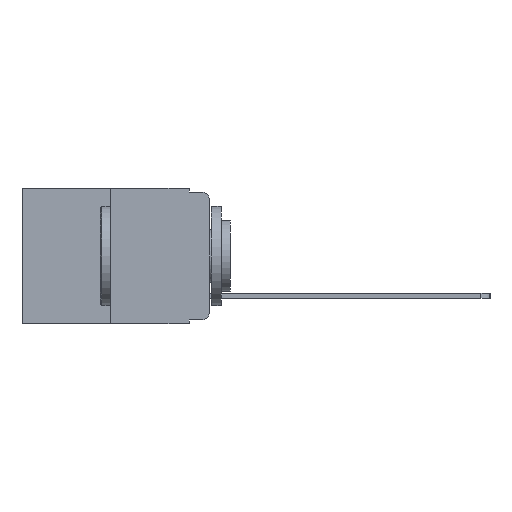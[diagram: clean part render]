
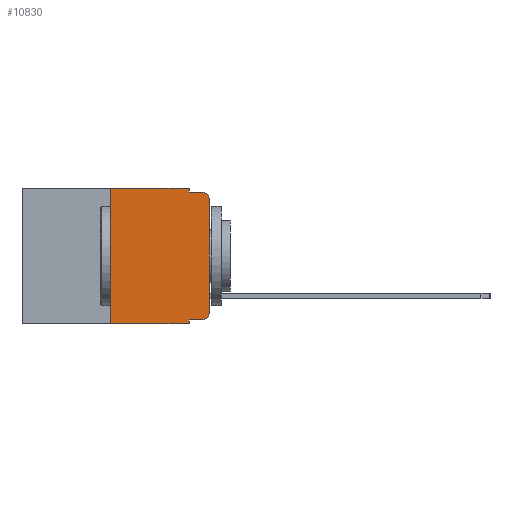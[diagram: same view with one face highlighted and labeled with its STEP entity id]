
A CAD part, left-side view. The second image highlights one B-rep face of the part: STEP entity #10830.
In plain terms, the highlighted planar face has unit normal (-1, 0, 0).
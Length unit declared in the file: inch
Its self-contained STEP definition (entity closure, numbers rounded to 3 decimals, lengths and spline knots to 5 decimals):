
#8 = CARTESIAN_POINT ( 'NONE',  ( 0., 0.051, 0. ) ) ;
#132 = CARTESIAN_POINT ( 'NONE',  ( 0., 0.25, -0.343 ) ) ;
#221 = VERTEX_POINT ( 'NONE', #3961 ) ;
#240 = LINE ( 'NONE', #15328, #3364 ) ;
#685 = VERTEX_POINT ( 'NONE', #11885 ) ;
#1372 = CARTESIAN_POINT ( 'NONE',  ( 0., 0.051, -0.01 ) ) ;
#1653 = ORIENTED_EDGE ( 'NONE', *, *, #17559, .T. ) ;
#2382 = VERTEX_POINT ( 'NONE', #10054 ) ;
#2571 = DIRECTION ( 'NONE',  ( 0., 0., -1. ) ) ;
#2594 = DIRECTION ( 'NONE',  ( 0., -1., 0. ) ) ;
#2757 = FACE_OUTER_BOUND ( 'NONE', #11270, .T. ) ;
#2986 = CARTESIAN_POINT ( 'NONE',  ( 0., 0.02, -0.313 ) ) ;
#3223 = DIRECTION ( 'NONE',  ( 0., 0., 1. ) ) ;
#3364 = VECTOR ( 'NONE', #18059, 39.37008 ) ;
#3961 = CARTESIAN_POINT ( 'NONE',  ( 0., 0., -0.313 ) ) ;
#4493 = DIRECTION ( 'NONE',  ( 0., 0., -1. ) ) ;
#4550 = VECTOR ( 'NONE', #17409, 39.37008 ) ;
#4647 = VERTEX_POINT ( 'NONE', #8 ) ;
#4823 = CARTESIAN_POINT ( 'NONE',  ( 0., 0.051, -0.333 ) ) ;
#5031 = CARTESIAN_POINT ( 'NONE',  ( 0., 0.473, 0. ) ) ;
#5142 = CIRCLE ( 'NONE', #14515, 0.02 ) ;
#5199 = VERTEX_POINT ( 'NONE', #7287 ) ;
#5489 = EDGE_CURVE ( 'NONE', #8750, #4647, #18431, .T. ) ;
#5506 = VECTOR ( 'NONE', #12727, 39.37008 ) ;
#5660 = ORIENTED_EDGE ( 'NONE', *, *, #14820, .F. ) ;
#6102 = ORIENTED_EDGE ( 'NONE', *, *, #5489, .F. ) ;
#6231 = CARTESIAN_POINT ( 'NONE',  ( 0., 0.051, 0. ) ) ;
#6409 = VERTEX_POINT ( 'NONE', #1372 ) ;
#6485 = LINE ( 'NONE', #9879, #17194 ) ;
#6561 = LINE ( 'NONE', #15604, #17689 ) ;
#6562 = ORIENTED_EDGE ( 'NONE', *, *, #12995, .F. ) ;
#6955 = VERTEX_POINT ( 'NONE', #4823 ) ;
#7062 = LINE ( 'NONE', #10476, #18149 ) ;
#7098 = CARTESIAN_POINT ( 'NONE',  ( 0., 0.25, 0. ) ) ;
#7259 = DIRECTION ( 'NONE',  ( -1., 0., 0. ) ) ;
#7287 = CARTESIAN_POINT ( 'NONE',  ( 0., 0., -0.03 ) ) ;
#7500 = ORIENTED_EDGE ( 'NONE', *, *, #9250, .T. ) ;
#7564 = VERTEX_POINT ( 'NONE', #132 ) ;
#8093 = CIRCLE ( 'NONE', #16236, 0.02 ) ;
#8441 = LINE ( 'NONE', #6231, #4550 ) ;
#8595 = AXIS2_PLACEMENT_3D ( 'NONE', #9854, #11267, #2571 ) ;
#8750 = VERTEX_POINT ( 'NONE', #10559 ) ;
#9063 = ORIENTED_EDGE ( 'NONE', *, *, #18463, .T. ) ;
#9250 = EDGE_CURVE ( 'NONE', #2382, #221, #8093, .T. ) ;
#9365 = LINE ( 'NONE', #7098, #5506 ) ;
#9854 = CARTESIAN_POINT ( 'NONE',  ( 0., 0.473, 0. ) ) ;
#9879 = CARTESIAN_POINT ( 'NONE',  ( 0., 0.051, -0.333 ) ) ;
#10054 = CARTESIAN_POINT ( 'NONE',  ( 0., 0.02, -0.333 ) ) ;
#10202 = EDGE_CURVE ( 'NONE', #6955, #2382, #6485, .T. ) ;
#10476 = CARTESIAN_POINT ( 'NONE',  ( 0., 0., 0. ) ) ;
#10559 = CARTESIAN_POINT ( 'NONE',  ( 0., 0.25, 0. ) ) ;
#10817 = ORIENTED_EDGE ( 'NONE', *, *, #10202, .T. ) ;
#10830 = ADVANCED_FACE ( 'NONE', ( #2757 ), #12592, .F. ) ;
#11126 = VECTOR ( 'NONE', #13601, 39.37008 ) ;
#11267 = DIRECTION ( 'NONE',  ( 1., 0., 0. ) ) ;
#11270 = EDGE_LOOP ( 'NONE', ( #9063, #1653, #5660, #16848, #6102, #6562, #14077, #17690, #10817, #7500 ) ) ;
#11885 = CARTESIAN_POINT ( 'NONE',  ( 0., 0.02, -0.01 ) ) ;
#12034 = EDGE_CURVE ( 'NONE', #6955, #14273, #17162, .T. ) ;
#12592 = PLANE ( 'NONE',  #8595 ) ;
#12727 = DIRECTION ( 'NONE',  ( 0., 0., 1. ) ) ;
#12995 = EDGE_CURVE ( 'NONE', #7564, #8750, #9365, .T. ) ;
#13060 = DIRECTION ( 'NONE',  ( -1., 0., 0. ) ) ;
#13540 = VECTOR ( 'NONE', #17748, 39.37008 ) ;
#13601 = DIRECTION ( 'NONE',  ( 0., -1., 0. ) ) ;
#13902 = EDGE_CURVE ( 'NONE', #4647, #6409, #8441, .T. ) ;
#14077 = ORIENTED_EDGE ( 'NONE', *, *, #14148, .T. ) ;
#14148 = EDGE_CURVE ( 'NONE', #7564, #14273, #240, .T. ) ;
#14273 = VERTEX_POINT ( 'NONE', #15686 ) ;
#14515 = AXIS2_PLACEMENT_3D ( 'NONE', #15633, #7259, #16993 ) ;
#14820 = EDGE_CURVE ( 'NONE', #6409, #685, #6561, .T. ) ;
#15328 = CARTESIAN_POINT ( 'NONE',  ( 0., 0.473, -0.343 ) ) ;
#15604 = CARTESIAN_POINT ( 'NONE',  ( 0., 0.051, -0.01 ) ) ;
#15633 = CARTESIAN_POINT ( 'NONE',  ( 0., 0.02, -0.03 ) ) ;
#15686 = CARTESIAN_POINT ( 'NONE',  ( 0., 0.051, -0.343 ) ) ;
#16236 = AXIS2_PLACEMENT_3D ( 'NONE', #2986, #13060, #4493 ) ;
#16386 = CARTESIAN_POINT ( 'NONE',  ( 0., 0.051, 0. ) ) ;
#16848 = ORIENTED_EDGE ( 'NONE', *, *, #13902, .F. ) ;
#16971 = DIRECTION ( 'NONE',  ( 0., -1., 0. ) ) ;
#16993 = DIRECTION ( 'NONE',  ( 0., 0., -1. ) ) ;
#17162 = LINE ( 'NONE', #16386, #13540 ) ;
#17194 = VECTOR ( 'NONE', #2594, 39.37008 ) ;
#17409 = DIRECTION ( 'NONE',  ( 0., 0., -1. ) ) ;
#17559 = EDGE_CURVE ( 'NONE', #5199, #685, #5142, .T. ) ;
#17689 = VECTOR ( 'NONE', #16971, 39.37008 ) ;
#17690 = ORIENTED_EDGE ( 'NONE', *, *, #12034, .F. ) ;
#17748 = DIRECTION ( 'NONE',  ( 0., 0., -1. ) ) ;
#18059 = DIRECTION ( 'NONE',  ( 0., -1., 0. ) ) ;
#18149 = VECTOR ( 'NONE', #3223, 39.37008 ) ;
#18431 = LINE ( 'NONE', #5031, #11126 ) ;
#18463 = EDGE_CURVE ( 'NONE', #221, #5199, #7062, .T. ) ;
